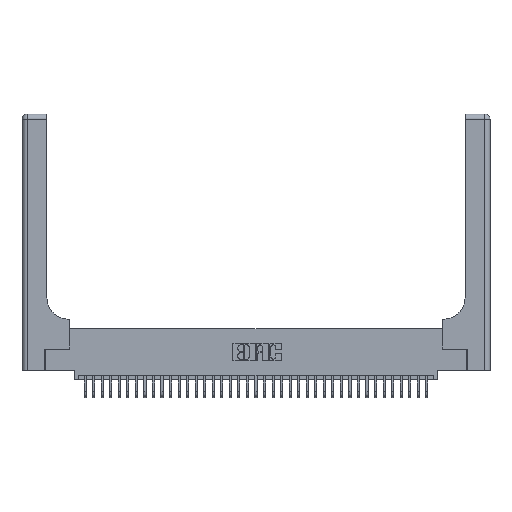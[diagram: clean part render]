
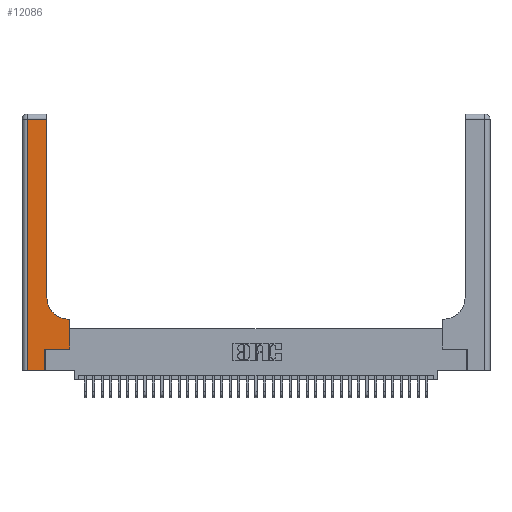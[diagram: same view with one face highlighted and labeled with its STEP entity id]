
A CAD part, top view. The second image highlights one B-rep face of the part: STEP entity #12086.
In plain terms, the highlighted planar face has unit normal (0, 0, 1).
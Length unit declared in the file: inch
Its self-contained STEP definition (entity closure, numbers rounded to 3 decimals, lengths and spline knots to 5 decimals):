
#229 = CARTESIAN_POINT ( 'NONE',  ( 0.06, 2.94, 0.37 ) ) ;
#1211 = AXIS2_PLACEMENT_3D ( 'NONE', #11920, #32891, #14927 ) ;
#1713 = LINE ( 'NONE', #23111, #31256 ) ;
#1729 = CARTESIAN_POINT ( 'NONE',  ( 0.5585, 0.25, 0.37 ) ) ;
#2051 = DIRECTION ( 'NONE',  ( 0., 1., 0. ) ) ;
#2887 = VECTOR ( 'NONE', #13051, 39.37008 ) ;
#5607 = VERTEX_POINT ( 'NONE', #17425 ) ;
#5798 = CIRCLE ( 'NONE', #34827, 0.25 ) ;
#5833 = ORIENTED_EDGE ( 'NONE', *, *, #21581, .T. ) ;
#6363 = CARTESIAN_POINT ( 'NONE',  ( 0.269, 0.25, 0.37 ) ) ;
#6675 = CARTESIAN_POINT ( 'NONE',  ( 0.2915, 0.6, 0.37 ) ) ;
#7786 = ORIENTED_EDGE ( 'NONE', *, *, #8805, .T. ) ;
#7830 = ORIENTED_EDGE ( 'NONE', *, *, #21121, .T. ) ;
#8395 = CARTESIAN_POINT ( 'NONE',  ( 0.269, 0., 0.37 ) ) ;
#8805 = EDGE_CURVE ( 'NONE', #38699, #31570, #30906, .T. ) ;
#9462 = VERTEX_POINT ( 'NONE', #6363 ) ;
#9963 = CARTESIAN_POINT ( 'NONE',  ( 0., 2.94, 0.37 ) ) ;
#10209 = ORIENTED_EDGE ( 'NONE', *, *, #11218, .T. ) ;
#10516 = VERTEX_POINT ( 'NONE', #13991 ) ;
#11218 = EDGE_CURVE ( 'NONE', #5607, #11235, #1713, .T. ) ;
#11235 = VERTEX_POINT ( 'NONE', #26205 ) ;
#11920 = CARTESIAN_POINT ( 'NONE',  ( 0., 3., 0.37 ) ) ;
#12086 = ADVANCED_FACE ( 'NONE', ( #35835 ), #14792, .F. ) ;
#12311 = VECTOR ( 'NONE', #22160, 39.37008 ) ;
#12539 = VERTEX_POINT ( 'NONE', #1729 ) ;
#13051 = DIRECTION ( 'NONE',  ( -1., 0., 0. ) ) ;
#13143 = CARTESIAN_POINT ( 'NONE',  ( 0.5585, 0.25, 0.37 ) ) ;
#13237 = LINE ( 'NONE', #13143, #12311 ) ;
#13671 = EDGE_CURVE ( 'NONE', #12539, #38699, #13237, .T. ) ;
#13991 = CARTESIAN_POINT ( 'NONE',  ( 0.2915, 0.85, 0.37 ) ) ;
#14792 = PLANE ( 'NONE',  #1211 ) ;
#14927 = DIRECTION ( 'NONE',  ( -1., 0., 0. ) ) ;
#15048 = EDGE_CURVE ( 'NONE', #27089, #21681, #27280, .T. ) ;
#15230 = CARTESIAN_POINT ( 'NONE',  ( 0.06, 3., 0.37 ) ) ;
#15688 = CARTESIAN_POINT ( 'NONE',  ( 0.2915, 3., 0.37 ) ) ;
#15798 = CARTESIAN_POINT ( 'NONE',  ( 0.2915, 2.94, 0.37 ) ) ;
#16552 = EDGE_CURVE ( 'NONE', #21681, #5607, #25627, .T. ) ;
#16844 = CARTESIAN_POINT ( 'NONE',  ( 0.5415, 0.85, 0.37 ) ) ;
#17425 = CARTESIAN_POINT ( 'NONE',  ( 0.06, 0., 0.37 ) ) ;
#18133 = LINE ( 'NONE', #24369, #33145 ) ;
#18173 = LINE ( 'NONE', #15688, #33181 ) ;
#18692 = DIRECTION ( 'NONE',  ( 0., 1., 0. ) ) ;
#19178 = ORIENTED_EDGE ( 'NONE', *, *, #38027, .T. ) ;
#19840 = DIRECTION ( 'NONE',  ( 1., 0., 0. ) ) ;
#20094 = DIRECTION ( 'NONE',  ( 1., 0., 0. ) ) ;
#20285 = LINE ( 'NONE', #8395, #35258 ) ;
#21121 = EDGE_CURVE ( 'NONE', #10516, #27089, #18173, .T. ) ;
#21581 = EDGE_CURVE ( 'NONE', #9462, #12539, #18133, .T. ) ;
#21681 = VERTEX_POINT ( 'NONE', #229 ) ;
#21956 = VECTOR ( 'NONE', #30854, 39.37008 ) ;
#22160 = DIRECTION ( 'NONE',  ( 0., 1., 0. ) ) ;
#23111 = CARTESIAN_POINT ( 'NONE',  ( 0., 0., 0.37 ) ) ;
#23947 = ORIENTED_EDGE ( 'NONE', *, *, #15048, .T. ) ;
#23966 = CARTESIAN_POINT ( 'NONE',  ( 0.5585, 0.6, 0.37 ) ) ;
#24369 = CARTESIAN_POINT ( 'NONE',  ( 0.269, 0.25, 0.37 ) ) ;
#25387 = EDGE_CURVE ( 'NONE', #31570, #10516, #5798, .T. ) ;
#25627 = LINE ( 'NONE', #15230, #32602 ) ;
#26205 = CARTESIAN_POINT ( 'NONE',  ( 0.269, 0., 0.37 ) ) ;
#27089 = VERTEX_POINT ( 'NONE', #15798 ) ;
#27280 = LINE ( 'NONE', #9963, #2887 ) ;
#27432 = DIRECTION ( 'NONE',  ( 1., 0., 0. ) ) ;
#27579 = EDGE_LOOP ( 'NONE', ( #7830, #23947, #33257, #10209, #19178, #5833, #30937, #7786, #31851 ) ) ;
#30854 = DIRECTION ( 'NONE',  ( -1., 0., 0. ) ) ;
#30906 = LINE ( 'NONE', #6675, #21956 ) ;
#30937 = ORIENTED_EDGE ( 'NONE', *, *, #13671, .T. ) ;
#31256 = VECTOR ( 'NONE', #20094, 39.37008 ) ;
#31570 = VERTEX_POINT ( 'NONE', #33860 ) ;
#31851 = ORIENTED_EDGE ( 'NONE', *, *, #25387, .T. ) ;
#32602 = VECTOR ( 'NONE', #36303, 39.37008 ) ;
#32891 = DIRECTION ( 'NONE',  ( 0., 0., -1. ) ) ;
#33145 = VECTOR ( 'NONE', #27432, 39.37008 ) ;
#33181 = VECTOR ( 'NONE', #18692, 39.37008 ) ;
#33257 = ORIENTED_EDGE ( 'NONE', *, *, #16552, .T. ) ;
#33860 = CARTESIAN_POINT ( 'NONE',  ( 0.5415, 0.6, 0.37 ) ) ;
#34827 = AXIS2_PLACEMENT_3D ( 'NONE', #16844, #37767, #19840 ) ;
#35258 = VECTOR ( 'NONE', #2051, 39.37008 ) ;
#35835 = FACE_OUTER_BOUND ( 'NONE', #27579, .T. ) ;
#36303 = DIRECTION ( 'NONE',  ( 0., -1., 0. ) ) ;
#37767 = DIRECTION ( 'NONE',  ( 0., 0., -1. ) ) ;
#38027 = EDGE_CURVE ( 'NONE', #11235, #9462, #20285, .T. ) ;
#38699 = VERTEX_POINT ( 'NONE', #23966 ) ;
